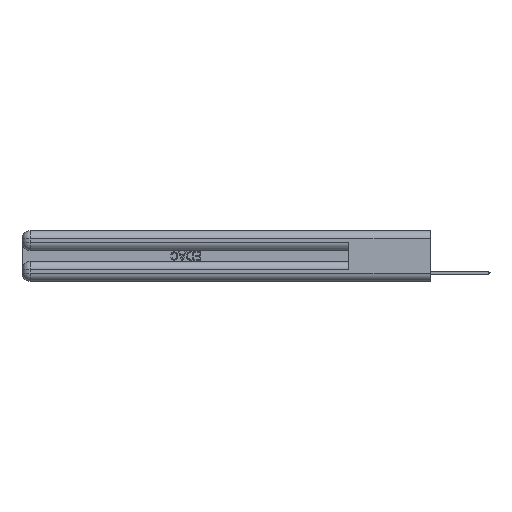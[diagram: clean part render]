
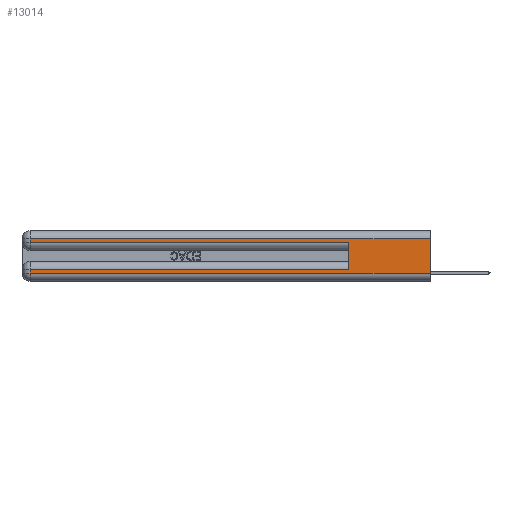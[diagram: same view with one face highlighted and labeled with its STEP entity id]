
A CAD part, left-side view. The second image highlights one B-rep face of the part: STEP entity #13014.
In plain terms, the highlighted planar face has unit normal (-1, 0, 0).
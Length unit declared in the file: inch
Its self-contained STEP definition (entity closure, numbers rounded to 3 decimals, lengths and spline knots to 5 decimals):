
#33 = VERTEX_POINT ( 'NONE', #2953 ) ;
#596 = AXIS2_PLACEMENT_3D ( 'NONE', #21075, #15213, #32071 ) ;
#710 = LINE ( 'NONE', #4559, #24234 ) ;
#1190 = DIRECTION ( 'NONE',  ( 0., 1., 0. ) ) ;
#1502 = VECTOR ( 'NONE', #27580, 39.37008 ) ;
#1760 = DIRECTION ( 'NONE',  ( 0., 0., -1. ) ) ;
#1898 = CARTESIAN_POINT ( 'NONE',  ( 0., 0.6, 0.285 ) ) ;
#2325 = LINE ( 'NONE', #13171, #8573 ) ;
#2953 = CARTESIAN_POINT ( 'NONE',  ( 0., 0.6, 0.085 ) ) ;
#3742 = CARTESIAN_POINT ( 'NONE',  ( 0., 2.94, 0.085 ) ) ;
#3833 = VECTOR ( 'NONE', #1190, 39.37008 ) ;
#3897 = ORIENTED_EDGE ( 'NONE', *, *, #24071, .T. ) ;
#4371 = LINE ( 'NONE', #12024, #3833 ) ;
#4426 = LINE ( 'NONE', #15266, #20153 ) ;
#4559 = CARTESIAN_POINT ( 'NONE',  ( 0., 0., 0.37 ) ) ;
#4985 = EDGE_CURVE ( 'NONE', #15454, #18620, #4426, .T. ) ;
#6265 = CARTESIAN_POINT ( 'NONE',  ( 0., 0., 0.31 ) ) ;
#6629 = VERTEX_POINT ( 'NONE', #1898 ) ;
#8562 = LINE ( 'NONE', #19416, #1502 ) ;
#8573 = VECTOR ( 'NONE', #24002, 39.37008 ) ;
#9427 = CARTESIAN_POINT ( 'NONE',  ( 0., 0., 0.06 ) ) ;
#9765 = VERTEX_POINT ( 'NONE', #22152 ) ;
#9874 = ORIENTED_EDGE ( 'NONE', *, *, #4985, .T. ) ;
#9955 = LINE ( 'NONE', #21170, #23423 ) ;
#10170 = ORIENTED_EDGE ( 'NONE', *, *, #12086, .T. ) ;
#10670 = CARTESIAN_POINT ( 'NONE',  ( 0., 2.94, 0.06 ) ) ;
#10744 = ORIENTED_EDGE ( 'NONE', *, *, #32975, .T. ) ;
#12024 = CARTESIAN_POINT ( 'NONE',  ( 0., 0., 0.31 ) ) ;
#12086 = EDGE_CURVE ( 'NONE', #18620, #9765, #33423, .T. ) ;
#12725 = DIRECTION ( 'NONE',  ( 0., 0., -1. ) ) ;
#13014 = ADVANCED_FACE ( 'NONE', ( #26056 ), #29226, .F. ) ;
#13171 = CARTESIAN_POINT ( 'NONE',  ( 0., 2.94, 0.37 ) ) ;
#13579 = EDGE_CURVE ( 'NONE', #15192, #31381, #2325, .T. ) ;
#15192 = VERTEX_POINT ( 'NONE', #18895 ) ;
#15213 = DIRECTION ( 'NONE',  ( 1., 0., 0. ) ) ;
#15266 = CARTESIAN_POINT ( 'NONE',  ( 0., 2.94, 0.37 ) ) ;
#15307 = DIRECTION ( 'NONE',  ( 0., 0., 1. ) ) ;
#15454 = VERTEX_POINT ( 'NONE', #3742 ) ;
#16957 = ORIENTED_EDGE ( 'NONE', *, *, #13579, .T. ) ;
#18426 = EDGE_CURVE ( 'NONE', #33, #6629, #9955, .T. ) ;
#18620 = VERTEX_POINT ( 'NONE', #10670 ) ;
#18715 = VECTOR ( 'NONE', #20626, 39.37008 ) ;
#18895 = CARTESIAN_POINT ( 'NONE',  ( 0., 2.94, 0.31 ) ) ;
#19115 = VECTOR ( 'NONE', #25449, 39.37008 ) ;
#19416 = CARTESIAN_POINT ( 'NONE',  ( 0., 0., 0.285 ) ) ;
#20153 = VECTOR ( 'NONE', #1760, 39.37008 ) ;
#20626 = DIRECTION ( 'NONE',  ( 0., -1., 0. ) ) ;
#21075 = CARTESIAN_POINT ( 'NONE',  ( 0., 0., 0.37 ) ) ;
#21170 = CARTESIAN_POINT ( 'NONE',  ( 0., 0.6, 0.145 ) ) ;
#22152 = CARTESIAN_POINT ( 'NONE',  ( 0., 0., 0.06 ) ) ;
#22607 = CARTESIAN_POINT ( 'NONE',  ( 0., 0., 0.085 ) ) ;
#23423 = VECTOR ( 'NONE', #15307, 39.37008 ) ;
#24002 = DIRECTION ( 'NONE',  ( 0., 0., -1. ) ) ;
#24071 = EDGE_CURVE ( 'NONE', #31381, #6629, #8562, .T. ) ;
#24234 = VECTOR ( 'NONE', #12725, 39.37008 ) ;
#24330 = ORIENTED_EDGE ( 'NONE', *, *, #33787, .T. ) ;
#24600 = ORIENTED_EDGE ( 'NONE', *, *, #18426, .F. ) ;
#25449 = DIRECTION ( 'NONE',  ( 0., 1., 0. ) ) ;
#26056 = FACE_OUTER_BOUND ( 'NONE', #33351, .T. ) ;
#27580 = DIRECTION ( 'NONE',  ( 0., -1., 0. ) ) ;
#29226 = PLANE ( 'NONE',  #596 ) ;
#29455 = CARTESIAN_POINT ( 'NONE',  ( 0., 2.94, 0.285 ) ) ;
#31381 = VERTEX_POINT ( 'NONE', #29455 ) ;
#32010 = ORIENTED_EDGE ( 'NONE', *, *, #34282, .F. ) ;
#32071 = DIRECTION ( 'NONE',  ( 0., 0., -1. ) ) ;
#32975 = EDGE_CURVE ( 'NONE', #34943, #15192, #4371, .T. ) ;
#33084 = LINE ( 'NONE', #22607, #19115 ) ;
#33351 = EDGE_LOOP ( 'NONE', ( #32010, #10744, #16957, #3897, #24600, #24330, #9874, #10170 ) ) ;
#33423 = LINE ( 'NONE', #9427, #18715 ) ;
#33787 = EDGE_CURVE ( 'NONE', #33, #15454, #33084, .T. ) ;
#34282 = EDGE_CURVE ( 'NONE', #34943, #9765, #710, .T. ) ;
#34943 = VERTEX_POINT ( 'NONE', #6265 ) ;
